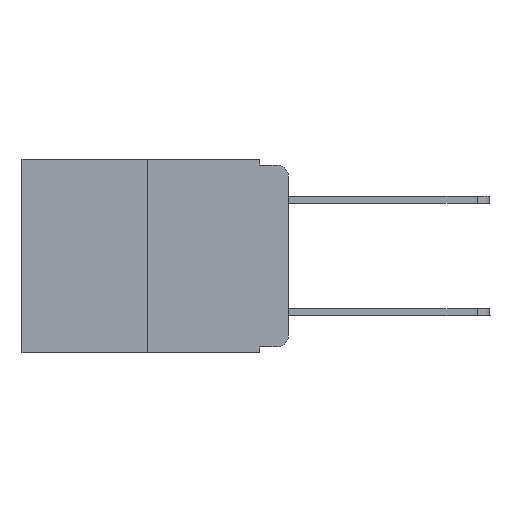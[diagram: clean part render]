
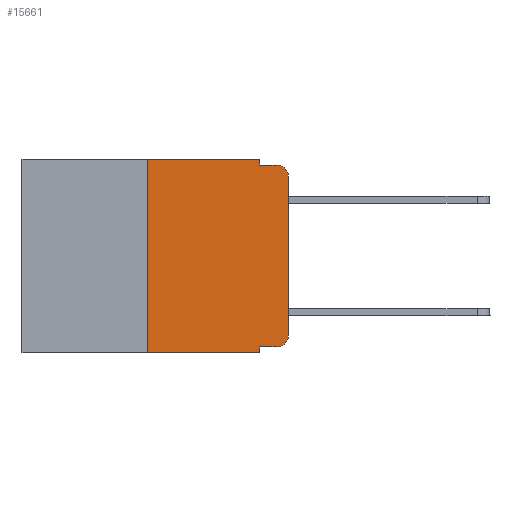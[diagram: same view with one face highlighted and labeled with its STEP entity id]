
A CAD part, left-side view. The second image highlights one B-rep face of the part: STEP entity #15661.
In plain terms, the highlighted planar face has unit normal (-1, 0, 0).
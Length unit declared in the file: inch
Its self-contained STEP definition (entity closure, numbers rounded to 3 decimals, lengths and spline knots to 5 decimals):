
#156 = ORIENTED_EDGE ( 'NONE', *, *, #12465, .F. ) ;
#922 = ORIENTED_EDGE ( 'NONE', *, *, #13434, .F. ) ;
#1118 = CARTESIAN_POINT ( 'NONE',  ( 0., 0.25, 0. ) ) ;
#1274 = CARTESIAN_POINT ( 'NONE',  ( 0., 0.051, -0.333 ) ) ;
#1709 = CARTESIAN_POINT ( 'NONE',  ( 0., 0.051, -0.01 ) ) ;
#1883 = VECTOR ( 'NONE', #7675, 39.37008 ) ;
#1937 = DIRECTION ( 'NONE',  ( 0., -1., 0. ) ) ;
#2275 = VECTOR ( 'NONE', #6943, 39.37008 ) ;
#2430 = DIRECTION ( 'NONE',  ( 0., 0., -1. ) ) ;
#2493 = VECTOR ( 'NONE', #17885, 39.37008 ) ;
#2818 = VERTEX_POINT ( 'NONE', #5731 ) ;
#3316 = VERTEX_POINT ( 'NONE', #7969 ) ;
#3380 = LINE ( 'NONE', #8310, #17212 ) ;
#3529 = CARTESIAN_POINT ( 'NONE',  ( 0., 0.02, -0.03 ) ) ;
#3701 = CARTESIAN_POINT ( 'NONE',  ( 0., 0.473, -0.343 ) ) ;
#3985 = EDGE_CURVE ( 'NONE', #14154, #2818, #11146, .T. ) ;
#3997 = LINE ( 'NONE', #19162, #13759 ) ;
#4242 = FACE_OUTER_BOUND ( 'NONE', #8587, .T. ) ;
#4373 = VECTOR ( 'NONE', #18330, 39.37008 ) ;
#4683 = AXIS2_PLACEMENT_3D ( 'NONE', #3529, #18790, #2430 ) ;
#5340 = CARTESIAN_POINT ( 'NONE',  ( 0., 0., -0.313 ) ) ;
#5731 = CARTESIAN_POINT ( 'NONE',  ( 0., 0., -0.03 ) ) ;
#5825 = AXIS2_PLACEMENT_3D ( 'NONE', #14190, #20708, #10923 ) ;
#6090 = EDGE_CURVE ( 'NONE', #3316, #14154, #12312, .T. ) ;
#6268 = LINE ( 'NONE', #8360, #11930 ) ;
#6403 = CARTESIAN_POINT ( 'NONE',  ( 0., 0.051, -0.343 ) ) ;
#6850 = ORIENTED_EDGE ( 'NONE', *, *, #6090, .T. ) ;
#6943 = DIRECTION ( 'NONE',  ( 0., -1., 0. ) ) ;
#7643 = CIRCLE ( 'NONE', #4683, 0.02 ) ;
#7675 = DIRECTION ( 'NONE',  ( 0., 0., 1. ) ) ;
#7764 = VERTEX_POINT ( 'NONE', #17524 ) ;
#7969 = CARTESIAN_POINT ( 'NONE',  ( 0., 0.02, -0.333 ) ) ;
#8001 = ORIENTED_EDGE ( 'NONE', *, *, #13461, .F. ) ;
#8169 = DIRECTION ( 'NONE',  ( 0., 0., 1. ) ) ;
#8310 = CARTESIAN_POINT ( 'NONE',  ( 0., 0.25, 0. ) ) ;
#8326 = CARTESIAN_POINT ( 'NONE',  ( 0., 0.051, -0.01 ) ) ;
#8360 = CARTESIAN_POINT ( 'NONE',  ( 0., 0.051, 0. ) ) ;
#8509 = CARTESIAN_POINT ( 'NONE',  ( 0., 0.473, 0. ) ) ;
#8587 = EDGE_LOOP ( 'NONE', ( #20677, #13998, #21175, #156, #922, #16777, #17037, #8001, #9582, #6850 ) ) ;
#9280 = PLANE ( 'NONE',  #5825 ) ;
#9582 = ORIENTED_EDGE ( 'NONE', *, *, #14464, .T. ) ;
#10194 = VERTEX_POINT ( 'NONE', #1274 ) ;
#10903 = DIRECTION ( 'NONE',  ( -1., 0., 0. ) ) ;
#10923 = DIRECTION ( 'NONE',  ( 0., 0., -1. ) ) ;
#11146 = LINE ( 'NONE', #17458, #1883 ) ;
#11390 = CARTESIAN_POINT ( 'NONE',  ( 0., 0.051, -0.333 ) ) ;
#11755 = EDGE_CURVE ( 'NONE', #2818, #7764, #7643, .T. ) ;
#11854 = LINE ( 'NONE', #8326, #4373 ) ;
#11930 = VECTOR ( 'NONE', #16913, 39.37008 ) ;
#12050 = LINE ( 'NONE', #3701, #2275 ) ;
#12312 = CIRCLE ( 'NONE', #14549, 0.02 ) ;
#12465 = EDGE_CURVE ( 'NONE', #16350, #16628, #3997, .T. ) ;
#13294 = LINE ( 'NONE', #11390, #2493 ) ;
#13434 = EDGE_CURVE ( 'NONE', #16986, #16350, #14988, .T. ) ;
#13461 = EDGE_CURVE ( 'NONE', #10194, #20706, #6268, .T. ) ;
#13759 = VECTOR ( 'NONE', #14005, 39.37008 ) ;
#13998 = ORIENTED_EDGE ( 'NONE', *, *, #11755, .T. ) ;
#14005 = DIRECTION ( 'NONE',  ( 0., 0., -1. ) ) ;
#14154 = VERTEX_POINT ( 'NONE', #5340 ) ;
#14190 = CARTESIAN_POINT ( 'NONE',  ( 0., 0.473, 0. ) ) ;
#14464 = EDGE_CURVE ( 'NONE', #10194, #3316, #13294, .T. ) ;
#14549 = AXIS2_PLACEMENT_3D ( 'NONE', #20979, #10903, #19256 ) ;
#14988 = LINE ( 'NONE', #8509, #17279 ) ;
#15661 = ADVANCED_FACE ( 'NONE', ( #4242 ), #9280, .F. ) ;
#16350 = VERTEX_POINT ( 'NONE', #20721 ) ;
#16628 = VERTEX_POINT ( 'NONE', #1709 ) ;
#16777 = ORIENTED_EDGE ( 'NONE', *, *, #17779, .F. ) ;
#16913 = DIRECTION ( 'NONE',  ( 0., 0., -1. ) ) ;
#16986 = VERTEX_POINT ( 'NONE', #1118 ) ;
#17037 = ORIENTED_EDGE ( 'NONE', *, *, #20194, .T. ) ;
#17212 = VECTOR ( 'NONE', #8169, 39.37008 ) ;
#17273 = CARTESIAN_POINT ( 'NONE',  ( 0., 0.25, -0.343 ) ) ;
#17279 = VECTOR ( 'NONE', #1937, 39.37008 ) ;
#17458 = CARTESIAN_POINT ( 'NONE',  ( 0., 0., 0. ) ) ;
#17524 = CARTESIAN_POINT ( 'NONE',  ( 0., 0.02, -0.01 ) ) ;
#17779 = EDGE_CURVE ( 'NONE', #21028, #16986, #3380, .T. ) ;
#17885 = DIRECTION ( 'NONE',  ( 0., -1., 0. ) ) ;
#18330 = DIRECTION ( 'NONE',  ( 0., -1., 0. ) ) ;
#18790 = DIRECTION ( 'NONE',  ( -1., 0., 0. ) ) ;
#19162 = CARTESIAN_POINT ( 'NONE',  ( 0., 0.051, 0. ) ) ;
#19174 = EDGE_CURVE ( 'NONE', #16628, #7764, #11854, .T. ) ;
#19256 = DIRECTION ( 'NONE',  ( 0., 0., -1. ) ) ;
#20194 = EDGE_CURVE ( 'NONE', #21028, #20706, #12050, .T. ) ;
#20677 = ORIENTED_EDGE ( 'NONE', *, *, #3985, .T. ) ;
#20706 = VERTEX_POINT ( 'NONE', #6403 ) ;
#20708 = DIRECTION ( 'NONE',  ( 1., 0., 0. ) ) ;
#20721 = CARTESIAN_POINT ( 'NONE',  ( 0., 0.051, 0. ) ) ;
#20979 = CARTESIAN_POINT ( 'NONE',  ( 0., 0.02, -0.313 ) ) ;
#21028 = VERTEX_POINT ( 'NONE', #17273 ) ;
#21175 = ORIENTED_EDGE ( 'NONE', *, *, #19174, .F. ) ;
